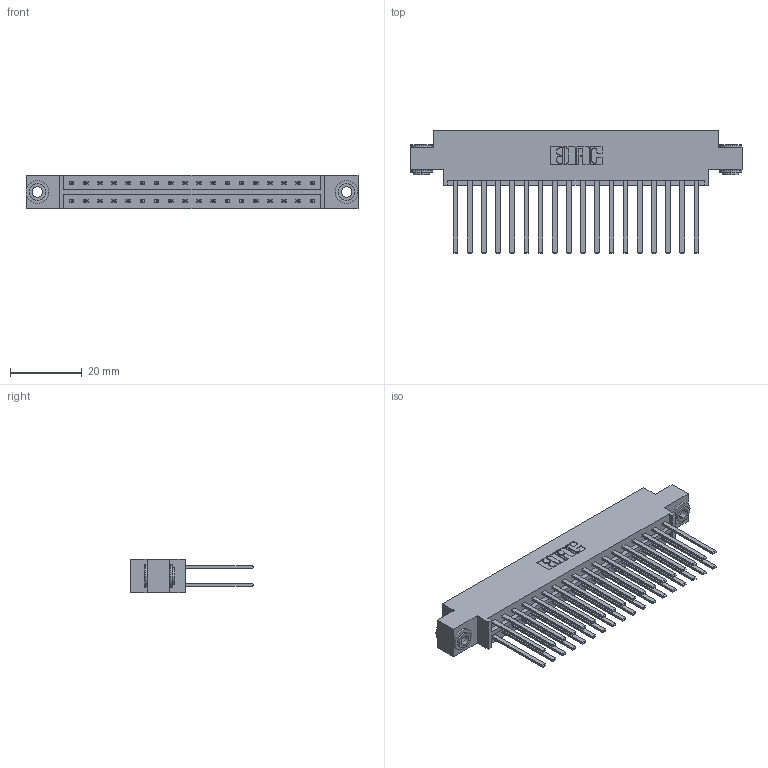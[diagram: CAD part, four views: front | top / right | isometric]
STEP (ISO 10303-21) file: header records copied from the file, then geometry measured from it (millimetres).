
FILE_DESCRIPTION (( 'STEP AP203' ), '1' );
FILE_NAME ('333-036-544-803.STEP', '2018-08-03T01:28:27', ( '' ), ( '' ), 'SwSTEP 2.0', 'SolidWorks 2016', '' );
FILE_SCHEMA (( 'CONFIG_CONTROL_DESIGN' ));
Length unit declared in the file: inch
Products named in the file (4): 333-036-544-803; 333 Part_Offset - .156 Dia - TH; 345-292-001_345-293-144; 345-250-002_345-250-002-102
Assembly tree (39 placements, depth 2):
  333-036-544-803
    333 Part_Offset - .156 Dia - TH
    345-292-001_345-293-144  x36
    345-250-002_345-250-002-102  x2
Bounding box: 92.86 x 34.3 x 9.4 mm (x, y, z)
Volume: 9552.5 mm3; surface area: 13102.2 mm2
Topology: 39 solids, 39 shells, 1812 faces, 5331 edges, 3502 vertices
Faces by surface type: plane 1236, cylinder 568, cone 8
Entity records: 15282 total; most frequent: CARTESIAN_POINT 2537, ORIENTED_EDGE 2466, DIRECTION 2239, EDGE_CURVE 1233, VECTOR 1085, LINE 1085, VERTEX_POINT 818, AXIS2_PLACEMENT_3D 577
